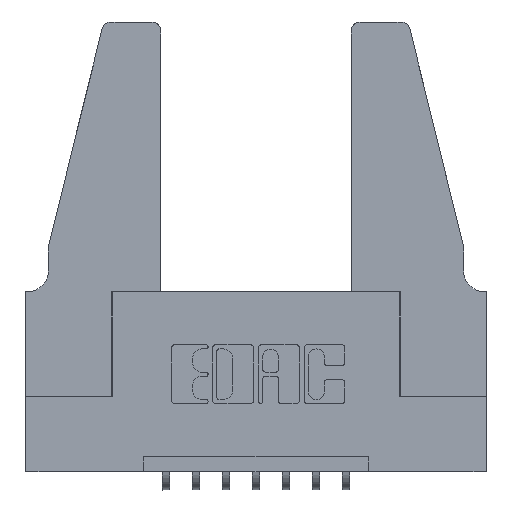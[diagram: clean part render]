
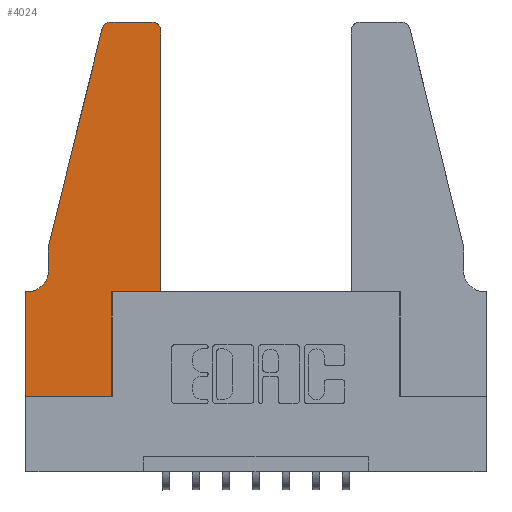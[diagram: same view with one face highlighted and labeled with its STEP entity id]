
A CAD part, top view. The second image highlights one B-rep face of the part: STEP entity #4024.
In plain terms, the highlighted planar face has unit normal (0, 0, 1).
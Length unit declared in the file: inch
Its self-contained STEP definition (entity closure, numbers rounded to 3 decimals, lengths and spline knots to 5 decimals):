
#61 = LINE ( 'NONE', #974, #2703 ) ;
#149 = VECTOR ( 'NONE', #8136, 39.37008 ) ;
#197 = CARTESIAN_POINT ( 'NONE',  ( 0.25487, 1.22718, 0.37 ) ) ;
#211 = LINE ( 'NONE', #8892, #1665 ) ;
#235 = CARTESIAN_POINT ( 'NONE',  ( 0.0755, 0.5, 0.37 ) ) ;
#302 = DIRECTION ( 'NONE',  ( 0., 0., 1. ) ) ;
#413 = VECTOR ( 'NONE', #10628, 39.37008 ) ;
#860 = VERTEX_POINT ( 'NONE', #197 ) ;
#903 = CARTESIAN_POINT ( 'NONE',  ( 0.0755, 0.42, 0.37 ) ) ;
#965 = CARTESIAN_POINT ( 'NONE',  ( 0., 0., 0.37 ) ) ;
#974 = CARTESIAN_POINT ( 'NONE',  ( 0.2865, 0.35, 0.37 ) ) ;
#995 = VERTEX_POINT ( 'NONE', #1189 ) ;
#1189 = CARTESIAN_POINT ( 'NONE',  ( 0.0055, 0.35, 0.37 ) ) ;
#1319 = EDGE_CURVE ( 'NONE', #9063, #6535, #7338, .T. ) ;
#1402 = LINE ( 'NONE', #10519, #9861 ) ;
#1665 = VECTOR ( 'NONE', #3112, 39.37008 ) ;
#1739 = EDGE_CURVE ( 'NONE', #5939, #860, #4819, .T. ) ;
#2090 = EDGE_CURVE ( 'NONE', #10603, #995, #3313, .T. ) ;
#2455 = ORIENTED_EDGE ( 'NONE', *, *, #5417, .T. ) ;
#2566 = ORIENTED_EDGE ( 'NONE', *, *, #9979, .T. ) ;
#2703 = VECTOR ( 'NONE', #10408, 39.37008 ) ;
#2836 = ORIENTED_EDGE ( 'NONE', *, *, #11332, .T. ) ;
#2864 = VECTOR ( 'NONE', #10324, 39.37008 ) ;
#2878 = EDGE_CURVE ( 'NONE', #4961, #5178, #5958, .T. ) ;
#2949 = EDGE_CURVE ( 'NONE', #6535, #5939, #3464, .T. ) ;
#3076 = EDGE_CURVE ( 'NONE', #5438, #11824, #211, .T. ) ;
#3085 = PLANE ( 'NONE',  #8006 ) ;
#3112 = DIRECTION ( 'NONE',  ( 1., 0., 0. ) ) ;
#3129 = ORIENTED_EDGE ( 'NONE', *, *, #2878, .T. ) ;
#3135 = CARTESIAN_POINT ( 'NONE',  ( 0.4505, 0.35, 0.37 ) ) ;
#3313 = CIRCLE ( 'NONE', #6073, 0.07 ) ;
#3392 = DIRECTION ( 'NONE',  ( 0., 0., 1. ) ) ;
#3464 = LINE ( 'NONE', #8546, #2864 ) ;
#3587 = VECTOR ( 'NONE', #4159, 39.37008 ) ;
#3639 = CARTESIAN_POINT ( 'NONE',  ( 0.4205, 1.22, 0.37 ) ) ;
#3724 = EDGE_CURVE ( 'NONE', #11824, #4961, #61, .T. ) ;
#4024 = ADVANCED_FACE ( 'NONE', ( #9973 ), #3085, .T. ) ;
#4159 = DIRECTION ( 'NONE',  ( 1., 0., 0. ) ) ;
#4369 = CARTESIAN_POINT ( 'NONE',  ( 0.4205, 1.25, 0.37 ) ) ;
#4776 = CARTESIAN_POINT ( 'NONE',  ( 0.0755, 0.5, 0.37 ) ) ;
#4777 = EDGE_CURVE ( 'NONE', #995, #11729, #10914, .T. ) ;
#4819 = CIRCLE ( 'NONE', #10281, 0.03 ) ;
#4961 = VERTEX_POINT ( 'NONE', #6769 ) ;
#5172 = DIRECTION ( 'NONE',  ( 1., 0., 0. ) ) ;
#5178 = VERTEX_POINT ( 'NONE', #10271 ) ;
#5289 = LINE ( 'NONE', #8714, #413 ) ;
#5293 = CARTESIAN_POINT ( 'NONE',  ( 0.0755, 0.35, 0.37 ) ) ;
#5296 = DIRECTION ( 'NONE',  ( 0., 0., -1. ) ) ;
#5417 = EDGE_CURVE ( 'NONE', #11729, #5438, #10466, .T. ) ;
#5438 = VERTEX_POINT ( 'NONE', #965 ) ;
#5497 = EDGE_LOOP ( 'NONE', ( #9732, #8123, #2566, #2836, #10884, #11952, #2455, #7057, #7247, #3129, #8959, #10144 ) ) ;
#5570 = CARTESIAN_POINT ( 'NONE',  ( 0.2865, 0., 0.37 ) ) ;
#5939 = VERTEX_POINT ( 'NONE', #11408 ) ;
#5958 = LINE ( 'NONE', #3135, #3587 ) ;
#6058 = CARTESIAN_POINT ( 'NONE',  ( 0.284, 1.22, 0.37 ) ) ;
#6073 = AXIS2_PLACEMENT_3D ( 'NONE', #10952, #5296, #7276 ) ;
#6535 = VERTEX_POINT ( 'NONE', #4369 ) ;
#6715 = CARTESIAN_POINT ( 'NONE',  ( 0., 0.35, 0.37 ) ) ;
#6769 = CARTESIAN_POINT ( 'NONE',  ( 0.2865, 0.35, 0.37 ) ) ;
#7057 = ORIENTED_EDGE ( 'NONE', *, *, #3076, .T. ) ;
#7247 = ORIENTED_EDGE ( 'NONE', *, *, #3724, .T. ) ;
#7276 = DIRECTION ( 'NONE',  ( -1., 0., 0. ) ) ;
#7338 = CIRCLE ( 'NONE', #10758, 0.03 ) ;
#7787 = DIRECTION ( 'NONE',  ( -0.239, -0.971, 0. ) ) ;
#8006 = AXIS2_PLACEMENT_3D ( 'NONE', #6715, #11428, #9642 ) ;
#8123 = ORIENTED_EDGE ( 'NONE', *, *, #1739, .T. ) ;
#8136 = DIRECTION ( 'NONE',  ( -1., 0., 0. ) ) ;
#8546 = CARTESIAN_POINT ( 'NONE',  ( 0.2605, 1.25, 0.37 ) ) ;
#8714 = CARTESIAN_POINT ( 'NONE',  ( 0.0755, 0.5, 0.37 ) ) ;
#8892 = CARTESIAN_POINT ( 'NONE',  ( 0., 0., 0.37 ) ) ;
#8959 = ORIENTED_EDGE ( 'NONE', *, *, #11563, .T. ) ;
#9063 = VERTEX_POINT ( 'NONE', #10886 ) ;
#9642 = DIRECTION ( 'NONE',  ( 1., 0., 0. ) ) ;
#9732 = ORIENTED_EDGE ( 'NONE', *, *, #2949, .T. ) ;
#9861 = VECTOR ( 'NONE', #10834, 39.37008 ) ;
#9973 = FACE_OUTER_BOUND ( 'NONE', #5497, .T. ) ;
#9979 = EDGE_CURVE ( 'NONE', #860, #10538, #10490, .T. ) ;
#10144 = ORIENTED_EDGE ( 'NONE', *, *, #1319, .T. ) ;
#10271 = CARTESIAN_POINT ( 'NONE',  ( 0.4505, 0.35, 0.37 ) ) ;
#10281 = AXIS2_PLACEMENT_3D ( 'NONE', #6058, #302, #5172 ) ;
#10321 = CARTESIAN_POINT ( 'NONE',  ( 0., 0., 0.37 ) ) ;
#10324 = DIRECTION ( 'NONE',  ( -1., 0., 0. ) ) ;
#10408 = DIRECTION ( 'NONE',  ( 0., 1., 0. ) ) ;
#10466 = LINE ( 'NONE', #10321, #10767 ) ;
#10490 = LINE ( 'NONE', #235, #11981 ) ;
#10519 = CARTESIAN_POINT ( 'NONE',  ( 0.4505, 0.35, 0.37 ) ) ;
#10538 = VERTEX_POINT ( 'NONE', #4776 ) ;
#10603 = VERTEX_POINT ( 'NONE', #903 ) ;
#10628 = DIRECTION ( 'NONE',  ( 0., -1., 0. ) ) ;
#10758 = AXIS2_PLACEMENT_3D ( 'NONE', #3639, #3392, #10909 ) ;
#10767 = VECTOR ( 'NONE', #11351, 39.37008 ) ;
#10834 = DIRECTION ( 'NONE',  ( 0., 1., 0. ) ) ;
#10884 = ORIENTED_EDGE ( 'NONE', *, *, #2090, .T. ) ;
#10886 = CARTESIAN_POINT ( 'NONE',  ( 0.4505, 1.22, 0.37 ) ) ;
#10909 = DIRECTION ( 'NONE',  ( 1., 0., 0. ) ) ;
#10914 = LINE ( 'NONE', #5293, #149 ) ;
#10952 = CARTESIAN_POINT ( 'NONE',  ( 0.0055, 0.42, 0.37 ) ) ;
#11115 = CARTESIAN_POINT ( 'NONE',  ( 0., 0.35, 0.37 ) ) ;
#11332 = EDGE_CURVE ( 'NONE', #10538, #10603, #5289, .T. ) ;
#11351 = DIRECTION ( 'NONE',  ( 0., -1., 0. ) ) ;
#11408 = CARTESIAN_POINT ( 'NONE',  ( 0.284, 1.25, 0.37 ) ) ;
#11428 = DIRECTION ( 'NONE',  ( 0., 0., 1. ) ) ;
#11563 = EDGE_CURVE ( 'NONE', #5178, #9063, #1402, .T. ) ;
#11729 = VERTEX_POINT ( 'NONE', #11115 ) ;
#11824 = VERTEX_POINT ( 'NONE', #5570 ) ;
#11952 = ORIENTED_EDGE ( 'NONE', *, *, #4777, .T. ) ;
#11981 = VECTOR ( 'NONE', #7787, 39.37008 ) ;
